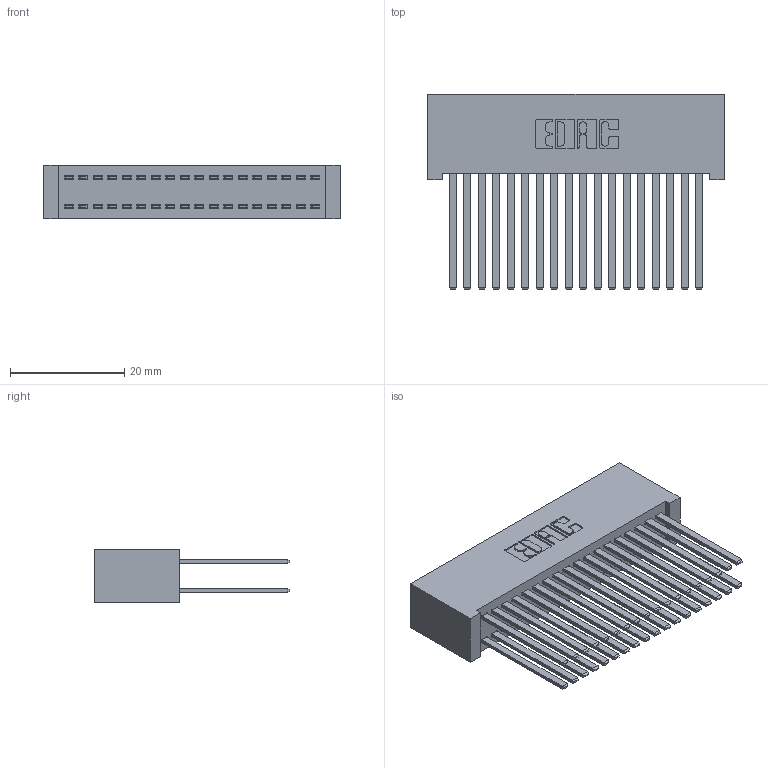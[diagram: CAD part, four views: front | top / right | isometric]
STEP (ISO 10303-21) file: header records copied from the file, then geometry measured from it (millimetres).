
FILE_DESCRIPTION (( 'STEP AP203' ), '1' );
FILE_NAME ('342-036-544-201.STEP', '2018-08-11T20:36:00', ( '' ), ( '' ), 'SwSTEP 2.0', 'SolidWorks 2016', '' );
FILE_SCHEMA (( 'CONFIG_CONTROL_DESIGN' ));
Length unit declared in the file: inch
Products named in the file (3): 342 Part_Lugless; 345-292-001_345-293-144; 342-036-544-201
Assembly tree (37 placements, depth 2):
  342-036-544-201
    342 Part_Lugless
    345-292-001_345-293-144  x36
Bounding box: 51.97 x 34.3 x 9.4 mm (x, y, z)
Volume: 5499.9 mm3; surface area: 10204.9 mm2
Topology: 37 solids, 37 shells, 1758 faces, 5207 edges, 3422 vertices
Faces by surface type: plane 1214, cylinder 544
Entity records: 14091 total; most frequent: CARTESIAN_POINT 2358, ORIENTED_EDGE 2294, DIRECTION 2047, EDGE_CURVE 1147, LINE 1031, VECTOR 1031, VERTEX_POINT 762, AXIS2_PLACEMENT_3D 508
